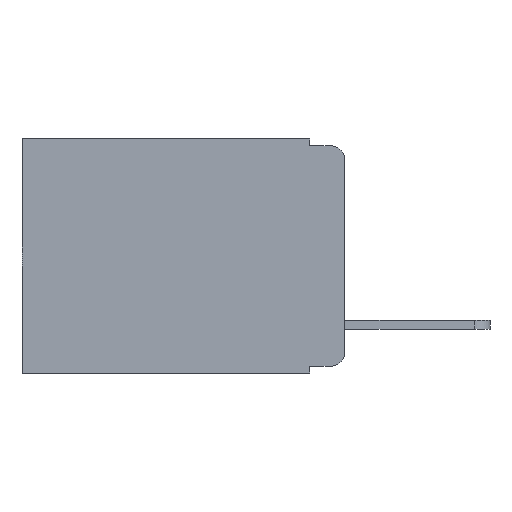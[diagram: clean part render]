
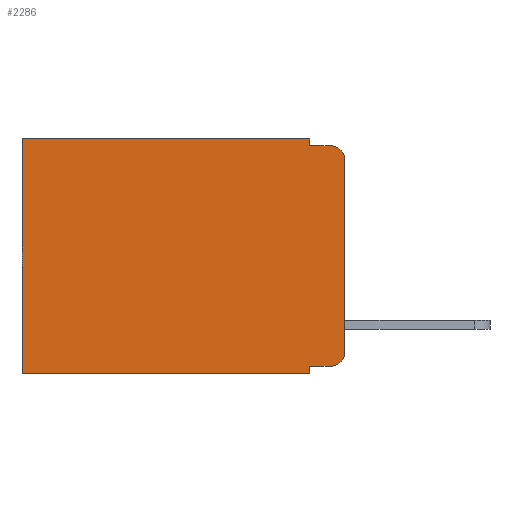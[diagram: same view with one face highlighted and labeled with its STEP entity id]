
A CAD part, left-side view. The second image highlights one B-rep face of the part: STEP entity #2286.
In plain terms, the highlighted planar face has unit normal (-1, 0, 0).
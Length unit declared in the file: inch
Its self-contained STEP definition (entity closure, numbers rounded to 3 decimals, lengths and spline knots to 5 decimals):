
#165 = CARTESIAN_POINT ( 'NONE',  ( 0.298, 0., 0. ) ) ;
#281 = CARTESIAN_POINT ( 'NONE',  ( 0.298, 0.051, -0.01 ) ) ;
#337 = EDGE_CURVE ( 'NONE', #8862, #1453, #7282, .T. ) ;
#363 = VERTEX_POINT ( 'NONE', #7993 ) ;
#900 = DIRECTION ( 'NONE',  ( 0., 0., -1. ) ) ;
#903 = DIRECTION ( 'NONE',  ( 0., 0., -1. ) ) ;
#933 = VERTEX_POINT ( 'NONE', #8056 ) ;
#1107 = EDGE_CURVE ( 'NONE', #1453, #363, #3904, .T. ) ;
#1156 = VERTEX_POINT ( 'NONE', #7301 ) ;
#1195 = CIRCLE ( 'NONE', #6553, 0.02 ) ;
#1375 = CARTESIAN_POINT ( 'NONE',  ( 0.298, 0., -0.313 ) ) ;
#1452 = EDGE_CURVE ( 'NONE', #10888, #6040, #4161, .T. ) ;
#1453 = VERTEX_POINT ( 'NONE', #8603 ) ;
#1557 = FACE_OUTER_BOUND ( 'NONE', #2988, .T. ) ;
#1766 = EDGE_CURVE ( 'NONE', #9946, #9749, #1195, .T. ) ;
#1939 = LINE ( 'NONE', #10837, #7904 ) ;
#2034 = DIRECTION ( 'NONE',  ( 0., 0., -1. ) ) ;
#2056 = DIRECTION ( 'NONE',  ( 0., 0., -1. ) ) ;
#2286 = ADVANCED_FACE ( 'NONE', ( #1557 ), #2957, .F. ) ;
#2354 = CARTESIAN_POINT ( 'NONE',  ( 0.298, 0.051, 0. ) ) ;
#2615 = DIRECTION ( 'NONE',  ( -1., 0., 0. ) ) ;
#2957 = PLANE ( 'NONE',  #4311 ) ;
#2988 = EDGE_LOOP ( 'NONE', ( #8329, #4399, #6330, #3934, #6647, #4222, #3762, #7811, #10460, #5836 ) ) ;
#3466 = CARTESIAN_POINT ( 'NONE',  ( 0.298, 0.02, -0.313 ) ) ;
#3612 = AXIS2_PLACEMENT_3D ( 'NONE', #7934, #2615, #8714 ) ;
#3760 = DIRECTION ( 'NONE',  ( 0., -1., 0. ) ) ;
#3762 = ORIENTED_EDGE ( 'NONE', *, *, #11299, .F. ) ;
#3892 = DIRECTION ( 'NONE',  ( 0., 1., 0. ) ) ;
#3904 = LINE ( 'NONE', #281, #9204 ) ;
#3909 = VECTOR ( 'NONE', #900, 39.37008 ) ;
#3934 = ORIENTED_EDGE ( 'NONE', *, *, #337, .F. ) ;
#4161 = LINE ( 'NONE', #2354, #7928 ) ;
#4222 = ORIENTED_EDGE ( 'NONE', *, *, #4496, .T. ) ;
#4311 = AXIS2_PLACEMENT_3D ( 'NONE', #165, #5534, #2034 ) ;
#4333 = CARTESIAN_POINT ( 'NONE',  ( 0.298, 0.051, 0. ) ) ;
#4399 = ORIENTED_EDGE ( 'NONE', *, *, #5453, .T. ) ;
#4496 = EDGE_CURVE ( 'NONE', #1156, #933, #5111, .T. ) ;
#5111 = LINE ( 'NONE', #8375, #11353 ) ;
#5210 = DIRECTION ( 'NONE',  ( 0., 0., -1. ) ) ;
#5453 = EDGE_CURVE ( 'NONE', #6079, #363, #8242, .T. ) ;
#5534 = DIRECTION ( 'NONE',  ( 1., 0., 0. ) ) ;
#5664 = DIRECTION ( 'NONE',  ( 0., 1., 0. ) ) ;
#5836 = ORIENTED_EDGE ( 'NONE', *, *, #1766, .T. ) ;
#5880 = EDGE_CURVE ( 'NONE', #6079, #9749, #9209, .T. ) ;
#6040 = VERTEX_POINT ( 'NONE', #8182 ) ;
#6043 = VECTOR ( 'NONE', #3892, 39.37008 ) ;
#6079 = VERTEX_POINT ( 'NONE', #8482 ) ;
#6330 = ORIENTED_EDGE ( 'NONE', *, *, #1107, .F. ) ;
#6532 = CARTESIAN_POINT ( 'NONE',  ( 0.298, 0., 0. ) ) ;
#6553 = AXIS2_PLACEMENT_3D ( 'NONE', #3466, #8803, #5210 ) ;
#6647 = ORIENTED_EDGE ( 'NONE', *, *, #9585, .T. ) ;
#7282 = LINE ( 'NONE', #4333, #11150 ) ;
#7301 = CARTESIAN_POINT ( 'NONE',  ( 0.298, 0.473, 0. ) ) ;
#7729 = LINE ( 'NONE', #9446, #9834 ) ;
#7811 = ORIENTED_EDGE ( 'NONE', *, *, #1452, .F. ) ;
#7904 = VECTOR ( 'NONE', #5664, 39.37008 ) ;
#7928 = VECTOR ( 'NONE', #9461, 39.37008 ) ;
#7934 = CARTESIAN_POINT ( 'NONE',  ( 0.298, 0.02, -0.03 ) ) ;
#7993 = CARTESIAN_POINT ( 'NONE',  ( 0.298, 0.02, -0.01 ) ) ;
#8056 = CARTESIAN_POINT ( 'NONE',  ( 0.298, 0.473, -0.343 ) ) ;
#8182 = CARTESIAN_POINT ( 'NONE',  ( 0.298, 0.051, -0.343 ) ) ;
#8242 = CIRCLE ( 'NONE', #3612, 0.02 ) ;
#8306 = CARTESIAN_POINT ( 'NONE',  ( 0.298, 0.051, -0.333 ) ) ;
#8329 = ORIENTED_EDGE ( 'NONE', *, *, #5880, .F. ) ;
#8375 = CARTESIAN_POINT ( 'NONE',  ( 0.298, 0.473, 0. ) ) ;
#8482 = CARTESIAN_POINT ( 'NONE',  ( 0.298, 0., -0.03 ) ) ;
#8603 = CARTESIAN_POINT ( 'NONE',  ( 0.298, 0.051, -0.01 ) ) ;
#8714 = DIRECTION ( 'NONE',  ( 0., 0., -1. ) ) ;
#8803 = DIRECTION ( 'NONE',  ( -1., 0., 0. ) ) ;
#8852 = CARTESIAN_POINT ( 'NONE',  ( 0.298, 0., 0. ) ) ;
#8862 = VERTEX_POINT ( 'NONE', #10442 ) ;
#9204 = VECTOR ( 'NONE', #3760, 39.37008 ) ;
#9209 = LINE ( 'NONE', #8852, #3909 ) ;
#9405 = EDGE_CURVE ( 'NONE', #10888, #9946, #7729, .T. ) ;
#9446 = CARTESIAN_POINT ( 'NONE',  ( 0.298, 0.051, -0.333 ) ) ;
#9461 = DIRECTION ( 'NONE',  ( 0., 0., -1. ) ) ;
#9585 = EDGE_CURVE ( 'NONE', #8862, #1156, #11469, .T. ) ;
#9749 = VERTEX_POINT ( 'NONE', #1375 ) ;
#9807 = CARTESIAN_POINT ( 'NONE',  ( 0.298, 0.02, -0.333 ) ) ;
#9834 = VECTOR ( 'NONE', #11291, 39.37008 ) ;
#9946 = VERTEX_POINT ( 'NONE', #9807 ) ;
#10442 = CARTESIAN_POINT ( 'NONE',  ( 0.298, 0.051, 0. ) ) ;
#10460 = ORIENTED_EDGE ( 'NONE', *, *, #9405, .T. ) ;
#10837 = CARTESIAN_POINT ( 'NONE',  ( 0.298, 0., -0.343 ) ) ;
#10888 = VERTEX_POINT ( 'NONE', #8306 ) ;
#11150 = VECTOR ( 'NONE', #903, 39.37008 ) ;
#11291 = DIRECTION ( 'NONE',  ( 0., -1., 0. ) ) ;
#11299 = EDGE_CURVE ( 'NONE', #6040, #933, #1939, .T. ) ;
#11353 = VECTOR ( 'NONE', #2056, 39.37008 ) ;
#11469 = LINE ( 'NONE', #6532, #6043 ) ;
